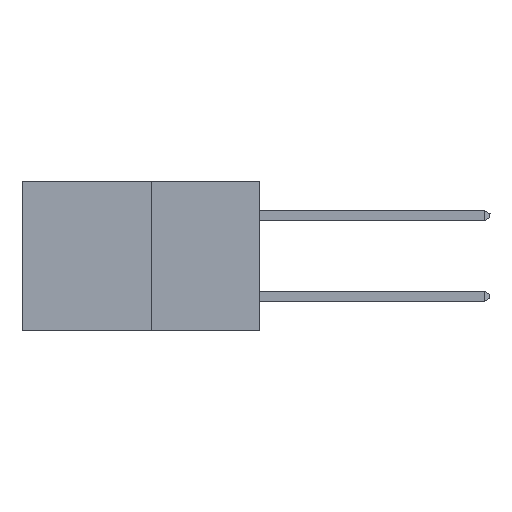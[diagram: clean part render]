
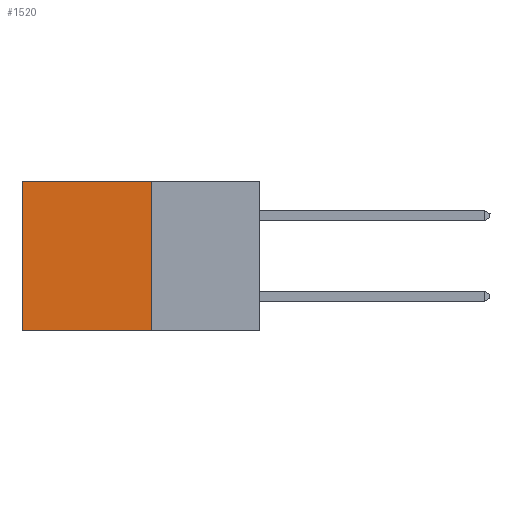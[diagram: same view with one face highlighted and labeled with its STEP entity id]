
A CAD part, left-side view. The second image highlights one B-rep face of the part: STEP entity #1520.
In plain terms, the highlighted planar face has unit normal (-1, 0, 0).
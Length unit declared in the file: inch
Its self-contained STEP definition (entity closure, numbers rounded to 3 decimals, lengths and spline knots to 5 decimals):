
#370 = EDGE_CURVE ( 'NONE', #7472, #12792, #10071, .T. ) ;
#376 = CARTESIAN_POINT ( 'NONE',  ( 0.277, 0.59, -0.37 ) ) ;
#570 = CARTESIAN_POINT ( 'NONE',  ( 0.277, 0.27, -0.37 ) ) ;
#1520 = ADVANCED_FACE ( 'NONE', ( #7589 ), #12492, .F. ) ;
#1635 = VECTOR ( 'NONE', #3406, 39.37008 ) ;
#1799 = EDGE_CURVE ( 'NONE', #7472, #10197, #1927, .T. ) ;
#1927 = LINE ( 'NONE', #2843, #9425 ) ;
#2120 = ORIENTED_EDGE ( 'NONE', *, *, #11801, .F. ) ;
#2504 = CARTESIAN_POINT ( 'NONE',  ( 0.277, 0.59, 0. ) ) ;
#2690 = LINE ( 'NONE', #376, #5426 ) ;
#2702 = CARTESIAN_POINT ( 'NONE',  ( 0.277, 0.27, -0.37 ) ) ;
#2843 = CARTESIAN_POINT ( 'NONE',  ( 0.277, 0.27, 0. ) ) ;
#3014 = VECTOR ( 'NONE', #10770, 39.37008 ) ;
#3091 = EDGE_LOOP ( 'NONE', ( #4970, #2120, #3968, #5301 ) ) ;
#3406 = DIRECTION ( 'NONE',  ( 0., 0., -1. ) ) ;
#3893 = AXIS2_PLACEMENT_3D ( 'NONE', #12172, #12065, #7029 ) ;
#3968 = ORIENTED_EDGE ( 'NONE', *, *, #370, .F. ) ;
#4970 = ORIENTED_EDGE ( 'NONE', *, *, #11376, .T. ) ;
#5301 = ORIENTED_EDGE ( 'NONE', *, *, #1799, .T. ) ;
#5426 = VECTOR ( 'NONE', #6601, 39.37008 ) ;
#6144 = DIRECTION ( 'NONE',  ( 0., 1., 0. ) ) ;
#6601 = DIRECTION ( 'NONE',  ( 0., 0., -1. ) ) ;
#7029 = DIRECTION ( 'NONE',  ( 0., 0., -1. ) ) ;
#7472 = VERTEX_POINT ( 'NONE', #9250 ) ;
#7589 = FACE_OUTER_BOUND ( 'NONE', #3091, .T. ) ;
#8677 = CARTESIAN_POINT ( 'NONE',  ( 0.277, 0.59, -0.37 ) ) ;
#9250 = CARTESIAN_POINT ( 'NONE',  ( 0.277, 0.27, 0. ) ) ;
#9425 = VECTOR ( 'NONE', #6144, 39.37008 ) ;
#10071 = LINE ( 'NONE', #2702, #1635 ) ;
#10197 = VERTEX_POINT ( 'NONE', #2504 ) ;
#10231 = VERTEX_POINT ( 'NONE', #8677 ) ;
#10735 = LINE ( 'NONE', #570, #3014 ) ;
#10770 = DIRECTION ( 'NONE',  ( 0., 1., 0. ) ) ;
#11376 = EDGE_CURVE ( 'NONE', #10197, #10231, #2690, .T. ) ;
#11801 = EDGE_CURVE ( 'NONE', #12792, #10231, #10735, .T. ) ;
#12065 = DIRECTION ( 'NONE',  ( 1., 0., 0. ) ) ;
#12172 = CARTESIAN_POINT ( 'NONE',  ( 0.277, 0.27, -0.37 ) ) ;
#12211 = CARTESIAN_POINT ( 'NONE',  ( 0.277, 0.27, -0.37 ) ) ;
#12492 = PLANE ( 'NONE',  #3893 ) ;
#12792 = VERTEX_POINT ( 'NONE', #12211 ) ;
